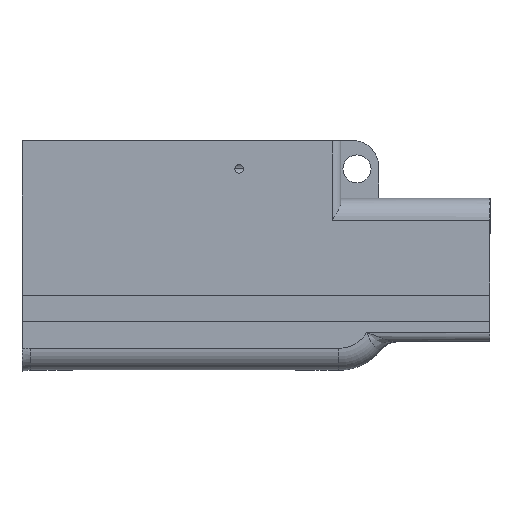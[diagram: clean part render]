
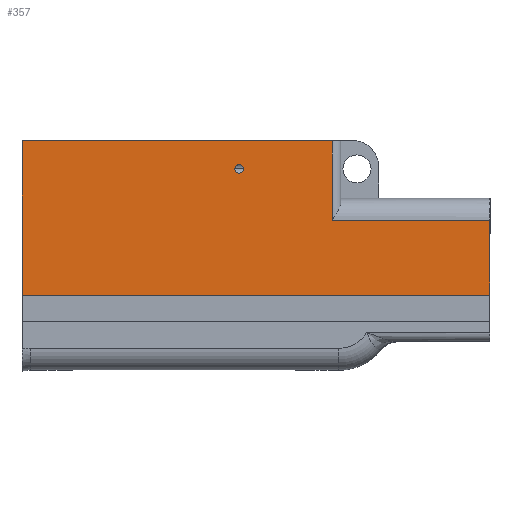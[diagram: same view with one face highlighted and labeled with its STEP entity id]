
A CAD part, top view. The second image highlights one B-rep face of the part: STEP entity #357.
In plain terms, the highlighted planar face has unit normal (0, 0, 1).
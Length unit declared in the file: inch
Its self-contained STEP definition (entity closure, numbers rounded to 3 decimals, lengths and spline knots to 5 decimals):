
#1 = VECTOR ( 'NONE', #422, 39.37008 ) ;
#11 = ORIENTED_EDGE ( 'NONE', *, *, #723, .T. ) ;
#29 = ORIENTED_EDGE ( 'NONE', *, *, #163, .T. ) ;
#34 = VECTOR ( 'NONE', #345, 39.37008 ) ;
#41 = ORIENTED_EDGE ( 'NONE', *, *, #171, .F. ) ;
#49 = CARTESIAN_POINT ( 'NONE',  ( -5.44519, -1.38086, 0.73097 ) ) ;
#73 = EDGE_CURVE ( 'NONE', #1393, #675, #685, .T. ) ;
#109 = VECTOR ( 'NONE', #863, 39.37008 ) ;
#155 = EDGE_CURVE ( 'NONE', #1393, #568, #861, .T. ) ;
#163 = EDGE_CURVE ( 'NONE', #282, #709, #1170, .T. ) ;
#171 = EDGE_CURVE ( 'NONE', #675, #709, #790, .T. ) ;
#178 = EDGE_CURVE ( 'NONE', #1591, #1617, #1479, .T. ) ;
#194 = VERTEX_POINT ( 'NONE', #460 ) ;
#271 = CARTESIAN_POINT ( 'NONE',  ( 3.70038, -0.47716, 0.73097 ) ) ;
#282 = VERTEX_POINT ( 'NONE', #1157 ) ;
#345 = DIRECTION ( 'NONE',  ( -1., 0., 0. ) ) ;
#357 = ADVANCED_FACE ( 'NONE', ( #1516, #1563 ), #467, .T. ) ;
#409 = VECTOR ( 'NONE', #1641, 39.37008 ) ;
#422 = DIRECTION ( 'NONE',  ( 0., 1., 0. ) ) ;
#449 = DIRECTION ( 'NONE',  ( 1., 0., 0. ) ) ;
#460 = CARTESIAN_POINT ( 'NONE',  ( 3.70038, -0.71157, 0.73097 ) ) ;
#466 = EDGE_LOOP ( 'NONE', ( #1463, #1030 ) ) ;
#467 = PLANE ( 'NONE',  #1088 ) ;
#544 = CARTESIAN_POINT ( 'NONE',  ( -0.49053, 0., 0.73097 ) ) ;
#568 = VERTEX_POINT ( 'NONE', #684 ) ;
#584 = CARTESIAN_POINT ( 'NONE',  ( -0.49053, -0.47716, 0.73097 ) ) ;
#613 = DIRECTION ( 'NONE',  ( 1., 0., 0. ) ) ;
#648 = AXIS2_PLACEMENT_3D ( 'NONE', #717, #1623, #842 ) ;
#649 = ORIENTED_EDGE ( 'NONE', *, *, #1697, .T. ) ;
#675 = VERTEX_POINT ( 'NONE', #544 ) ;
#684 = CARTESIAN_POINT ( 'NONE',  ( 3.70038, -1.38086, 0.73097 ) ) ;
#685 = LINE ( 'NONE', #584, #1 ) ;
#709 = VERTEX_POINT ( 'NONE', #957 ) ;
#717 = CARTESIAN_POINT ( 'NONE',  ( 1.4543, -0.2505, 0.73097 ) ) ;
#719 = VECTOR ( 'NONE', #1346, 39.37008 ) ;
#723 = EDGE_CURVE ( 'NONE', #568, #194, #1068, .T. ) ;
#739 = CARTESIAN_POINT ( 'NONE',  ( 2.28556, 0., 0.73097 ) ) ;
#745 = DIRECTION ( 'NONE',  ( 0., 0., -1. ) ) ;
#753 = CARTESIAN_POINT ( 'NONE',  ( -0.1955, -0.47716, 0.73097 ) ) ;
#790 = LINE ( 'NONE', #1513, #409 ) ;
#826 = VECTOR ( 'NONE', #449, 39.37008 ) ;
#842 = DIRECTION ( 'NONE',  ( 1., 0., 0. ) ) ;
#861 = LINE ( 'NONE', #49, #826 ) ;
#863 = DIRECTION ( 'NONE',  ( 0., 1., 0. ) ) ;
#957 = CARTESIAN_POINT ( 'NONE',  ( 2.28556, 0., 0.73097 ) ) ;
#990 = EDGE_LOOP ( 'NONE', ( #1546, #1083, #11, #649, #29, #41 ) ) ;
#1010 = CARTESIAN_POINT ( 'NONE',  ( 1.4543, -0.2115, 0.73097 ) ) ;
#1030 = ORIENTED_EDGE ( 'NONE', *, *, #178, .T. ) ;
#1068 = LINE ( 'NONE', #271, #719 ) ;
#1083 = ORIENTED_EDGE ( 'NONE', *, *, #155, .T. ) ;
#1088 = AXIS2_PLACEMENT_3D ( 'NONE', #753, #1398, #613 ) ;
#1122 = CARTESIAN_POINT ( 'NONE',  ( -0.49053, -1.38086, 0.73097 ) ) ;
#1138 = CARTESIAN_POINT ( 'NONE',  ( 1.4543, -0.2895, 0.73097 ) ) ;
#1157 = CARTESIAN_POINT ( 'NONE',  ( 2.28556, -0.71157, 0.73097 ) ) ;
#1170 = LINE ( 'NONE', #739, #109 ) ;
#1211 = AXIS2_PLACEMENT_3D ( 'NONE', #1515, #745, #1646 ) ;
#1334 = EDGE_CURVE ( 'NONE', #1617, #1591, #1647, .T. ) ;
#1346 = DIRECTION ( 'NONE',  ( 0., 1., 0. ) ) ;
#1393 = VERTEX_POINT ( 'NONE', #1122 ) ;
#1398 = DIRECTION ( 'NONE',  ( 0., 0., 1. ) ) ;
#1420 = CARTESIAN_POINT ( 'NONE',  ( 0.42738, -0.71157, 0.73097 ) ) ;
#1457 = LINE ( 'NONE', #1420, #34 ) ;
#1463 = ORIENTED_EDGE ( 'NONE', *, *, #1334, .T. ) ;
#1479 = CIRCLE ( 'NONE', #1211, 0.039 ) ;
#1513 = CARTESIAN_POINT ( 'NONE',  ( 2.5093, 0., 0.73097 ) ) ;
#1515 = CARTESIAN_POINT ( 'NONE',  ( 1.4543, -0.2505, 0.73097 ) ) ;
#1516 = FACE_OUTER_BOUND ( 'NONE', #990, .T. ) ;
#1546 = ORIENTED_EDGE ( 'NONE', *, *, #73, .F. ) ;
#1563 = FACE_BOUND ( 'NONE', #466, .T. ) ;
#1591 = VERTEX_POINT ( 'NONE', #1010 ) ;
#1617 = VERTEX_POINT ( 'NONE', #1138 ) ;
#1623 = DIRECTION ( 'NONE',  ( 0., 0., -1. ) ) ;
#1641 = DIRECTION ( 'NONE',  ( 1., 0., 0. ) ) ;
#1646 = DIRECTION ( 'NONE',  ( 1., 0., 0. ) ) ;
#1647 = CIRCLE ( 'NONE', #648, 0.039 ) ;
#1697 = EDGE_CURVE ( 'NONE', #194, #282, #1457, .T. ) ;
